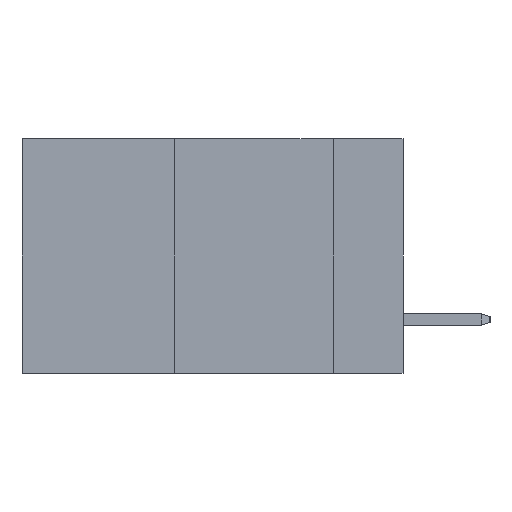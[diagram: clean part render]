
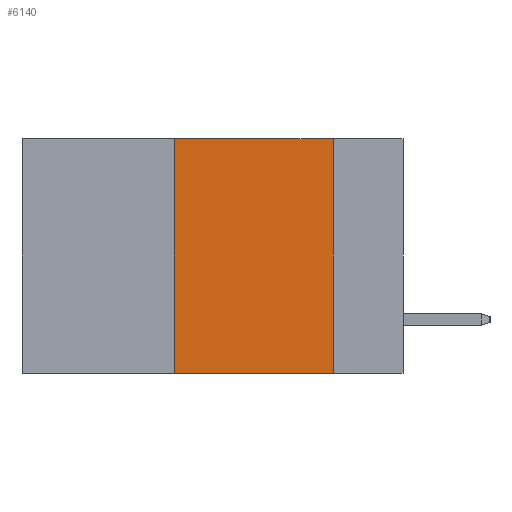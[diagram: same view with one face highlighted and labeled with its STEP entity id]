
A CAD part, left-side view. The second image highlights one B-rep face of the part: STEP entity #6140.
In plain terms, the highlighted planar face has unit normal (-1, 0, 0).
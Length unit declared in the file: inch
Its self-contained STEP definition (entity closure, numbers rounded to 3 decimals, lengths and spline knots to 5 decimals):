
#621 = DIRECTION ( 'NONE',  ( 0., 0., -1. ) ) ;
#897 = CARTESIAN_POINT ( 'NONE',  ( 0., 0.6, -0.37 ) ) ;
#1030 = VECTOR ( 'NONE', #7522, 39.37008 ) ;
#1286 = LINE ( 'NONE', #11268, #12535 ) ;
#1857 = VECTOR ( 'NONE', #11194, 39.37008 ) ;
#2057 = PLANE ( 'NONE',  #4841 ) ;
#2596 = CARTESIAN_POINT ( 'NONE',  ( 0., 0.11, 0. ) ) ;
#2851 = ORIENTED_EDGE ( 'NONE', *, *, #8779, .T. ) ;
#3132 = FACE_OUTER_BOUND ( 'NONE', #8160, .T. ) ;
#3475 = CARTESIAN_POINT ( 'NONE',  ( 0., 0.11, 0. ) ) ;
#4832 = CARTESIAN_POINT ( 'NONE',  ( 0., 0.36, 0. ) ) ;
#4841 = AXIS2_PLACEMENT_3D ( 'NONE', #9034, #8000, #7926 ) ;
#4862 = VERTEX_POINT ( 'NONE', #7154 ) ;
#4976 = ORIENTED_EDGE ( 'NONE', *, *, #9041, .F. ) ;
#4981 = ORIENTED_EDGE ( 'NONE', *, *, #9107, .F. ) ;
#5401 = CARTESIAN_POINT ( 'NONE',  ( 0., 0.11, -0.37 ) ) ;
#6140 = ADVANCED_FACE ( 'NONE', ( #3132 ), #2057, .F. ) ;
#7019 = VERTEX_POINT ( 'NONE', #2596 ) ;
#7154 = CARTESIAN_POINT ( 'NONE',  ( 0., 0.36, -0.37 ) ) ;
#7355 = LINE ( 'NONE', #3475, #9735 ) ;
#7450 = VERTEX_POINT ( 'NONE', #5401 ) ;
#7522 = DIRECTION ( 'NONE',  ( 0., -1., 0. ) ) ;
#7664 = ORIENTED_EDGE ( 'NONE', *, *, #12076, .F. ) ;
#7926 = DIRECTION ( 'NONE',  ( 0., 0., -1. ) ) ;
#7987 = VERTEX_POINT ( 'NONE', #4832 ) ;
#8000 = DIRECTION ( 'NONE',  ( 1., 0., 0. ) ) ;
#8160 = EDGE_LOOP ( 'NONE', ( #7664, #4976, #4981, #2851 ) ) ;
#8186 = CARTESIAN_POINT ( 'NONE',  ( 0., 0.6, 0. ) ) ;
#8779 = EDGE_CURVE ( 'NONE', #4862, #7450, #9543, .T. ) ;
#9034 = CARTESIAN_POINT ( 'NONE',  ( 0., 0.6, 0. ) ) ;
#9041 = EDGE_CURVE ( 'NONE', #7987, #7019, #9405, .T. ) ;
#9107 = EDGE_CURVE ( 'NONE', #4862, #7987, #1286, .T. ) ;
#9405 = LINE ( 'NONE', #8186, #1857 ) ;
#9543 = LINE ( 'NONE', #897, #1030 ) ;
#9735 = VECTOR ( 'NONE', #621, 39.37008 ) ;
#11194 = DIRECTION ( 'NONE',  ( 0., -1., 0. ) ) ;
#11268 = CARTESIAN_POINT ( 'NONE',  ( 0., 0.36, 0. ) ) ;
#12076 = EDGE_CURVE ( 'NONE', #7019, #7450, #7355, .T. ) ;
#12083 = DIRECTION ( 'NONE',  ( 0., 0., 1. ) ) ;
#12535 = VECTOR ( 'NONE', #12083, 39.37008 ) ;
